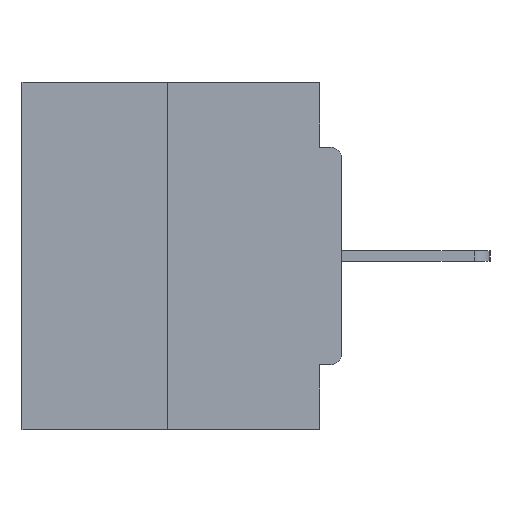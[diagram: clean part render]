
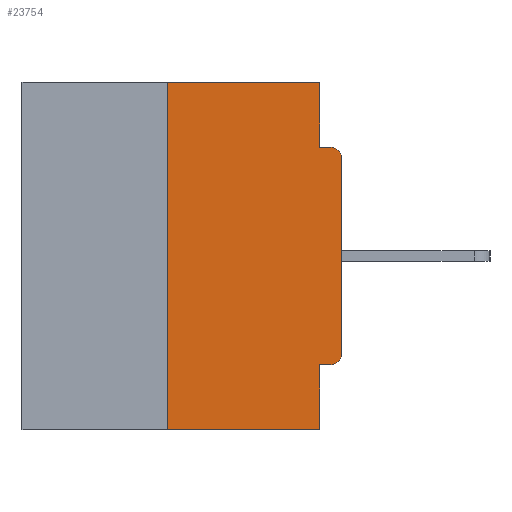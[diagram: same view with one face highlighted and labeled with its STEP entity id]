
A CAD part, left-side view. The second image highlights one B-rep face of the part: STEP entity #23754.
In plain terms, the highlighted planar face has unit normal (-1, 0, 0).
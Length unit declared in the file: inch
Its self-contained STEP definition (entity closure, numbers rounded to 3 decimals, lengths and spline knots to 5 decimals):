
#402 = VERTEX_POINT ( 'NONE', #31273 ) ;
#1106 = LINE ( 'NONE', #25379, #15881 ) ;
#1269 = VECTOR ( 'NONE', #26337, 39.37008 ) ;
#1753 = VERTEX_POINT ( 'NONE', #14833 ) ;
#2155 = VECTOR ( 'NONE', #20694, 39.37008 ) ;
#2261 = AXIS2_PLACEMENT_3D ( 'NONE', #11669, #24224, #5452 ) ;
#4445 = CARTESIAN_POINT ( 'NONE',  ( 0., 0., 0. ) ) ;
#5279 = CARTESIAN_POINT ( 'NONE',  ( 0., 0., -0.3915 ) ) ;
#5452 = DIRECTION ( 'NONE',  ( 0., 0., -1. ) ) ;
#5919 = EDGE_CURVE ( 'NONE', #8940, #1753, #33247, .T. ) ;
#6620 = DIRECTION ( 'NONE',  ( 0., 0., -1. ) ) ;
#6693 = CARTESIAN_POINT ( 'NONE',  ( 0., 0.015, -0.1085 ) ) ;
#6732 = ORIENTED_EDGE ( 'NONE', *, *, #8982, .T. ) ;
#8554 = VERTEX_POINT ( 'NONE', #39500 ) ;
#8940 = VERTEX_POINT ( 'NONE', #19826 ) ;
#8982 = EDGE_CURVE ( 'NONE', #19661, #14767, #25337, .T. ) ;
#9300 = VECTOR ( 'NONE', #33938, 39.37008 ) ;
#9754 = CARTESIAN_POINT ( 'NONE',  ( 0., 0., -0.1085 ) ) ;
#9851 = DIRECTION ( 'NONE',  ( 0., 0., -1. ) ) ;
#10511 = CARTESIAN_POINT ( 'NONE',  ( 0., 0.015, -0.0935 ) ) ;
#11559 = AXIS2_PLACEMENT_3D ( 'NONE', #17037, #38609, #20170 ) ;
#11669 = CARTESIAN_POINT ( 'NONE',  ( 0., 0.46, 0. ) ) ;
#12365 = CARTESIAN_POINT ( 'NONE',  ( 0., 0.46, -0.5 ) ) ;
#13371 = LINE ( 'NONE', #34215, #20705 ) ;
#14767 = VERTEX_POINT ( 'NONE', #9754 ) ;
#14833 = CARTESIAN_POINT ( 'NONE',  ( 0., 0.031, -0.5 ) ) ;
#15376 = DIRECTION ( 'NONE',  ( 0., -1., 0. ) ) ;
#15881 = VECTOR ( 'NONE', #6620, 39.37008 ) ;
#17037 = CARTESIAN_POINT ( 'NONE',  ( 0., 0.015, -0.3915 ) ) ;
#17578 = CARTESIAN_POINT ( 'NONE',  ( 0., 0., -0.4065 ) ) ;
#19661 = VERTEX_POINT ( 'NONE', #5279 ) ;
#19826 = CARTESIAN_POINT ( 'NONE',  ( 0., 0.031, -0.4065 ) ) ;
#20170 = DIRECTION ( 'NONE',  ( 0., 0., -1. ) ) ;
#20490 = VECTOR ( 'NONE', #21848, 39.37008 ) ;
#20694 = DIRECTION ( 'NONE',  ( 0., 1., 0. ) ) ;
#20705 = VECTOR ( 'NONE', #21890, 39.37008 ) ;
#21716 = ORIENTED_EDGE ( 'NONE', *, *, #23352, .F. ) ;
#21848 = DIRECTION ( 'NONE',  ( 0., 0., -1. ) ) ;
#21890 = DIRECTION ( 'NONE',  ( 0., -1., 0. ) ) ;
#22040 = ORIENTED_EDGE ( 'NONE', *, *, #30356, .F. ) ;
#22566 = ORIENTED_EDGE ( 'NONE', *, *, #37879, .T. ) ;
#22876 = LINE ( 'NONE', #34793, #38276 ) ;
#23080 = ORIENTED_EDGE ( 'NONE', *, *, #5919, .F. ) ;
#23352 = EDGE_CURVE ( 'NONE', #402, #8554, #22876, .T. ) ;
#23379 = ORIENTED_EDGE ( 'NONE', *, *, #26180, .T. ) ;
#23754 = ADVANCED_FACE ( 'NONE', ( #40130 ), #39527, .F. ) ;
#23858 = VECTOR ( 'NONE', #15376, 39.37008 ) ;
#24168 = VERTEX_POINT ( 'NONE', #38829 ) ;
#24224 = DIRECTION ( 'NONE',  ( 1., 0., 0. ) ) ;
#24860 = ORIENTED_EDGE ( 'NONE', *, *, #25760, .T. ) ;
#25337 = LINE ( 'NONE', #4445, #1269 ) ;
#25379 = CARTESIAN_POINT ( 'NONE',  ( 0., 0.031, 0. ) ) ;
#25760 = EDGE_CURVE ( 'NONE', #24168, #19661, #38092, .T. ) ;
#26069 = CIRCLE ( 'NONE', #33727, 0.015 ) ;
#26111 = EDGE_CURVE ( 'NONE', #35711, #40118, #13371, .T. ) ;
#26180 = EDGE_CURVE ( 'NONE', #14767, #40118, #26069, .T. ) ;
#26337 = DIRECTION ( 'NONE',  ( 0., 0., 1. ) ) ;
#26471 = CARTESIAN_POINT ( 'NONE',  ( 0., 0.25, -0.5 ) ) ;
#26864 = VERTEX_POINT ( 'NONE', #26471 ) ;
#27866 = LINE ( 'NONE', #30844, #9300 ) ;
#28027 = ORIENTED_EDGE ( 'NONE', *, *, #26111, .F. ) ;
#28565 = DIRECTION ( 'NONE',  ( -1., 0., 0. ) ) ;
#28619 = DIRECTION ( 'NONE',  ( 0., -1., 0. ) ) ;
#29087 = ORIENTED_EDGE ( 'NONE', *, *, #36549, .F. ) ;
#29676 = CARTESIAN_POINT ( 'NONE',  ( 0., 0.031, -0.0935 ) ) ;
#30356 = EDGE_CURVE ( 'NONE', #24168, #8940, #33422, .T. ) ;
#30844 = CARTESIAN_POINT ( 'NONE',  ( 0., 0.25, 0. ) ) ;
#31273 = CARTESIAN_POINT ( 'NONE',  ( 0., 0.25, 0. ) ) ;
#33247 = LINE ( 'NONE', #37211, #20490 ) ;
#33422 = LINE ( 'NONE', #17578, #2155 ) ;
#33727 = AXIS2_PLACEMENT_3D ( 'NONE', #6693, #28565, #9851 ) ;
#33938 = DIRECTION ( 'NONE',  ( 0., 0., 1. ) ) ;
#34215 = CARTESIAN_POINT ( 'NONE',  ( 0., 0., -0.0935 ) ) ;
#34494 = EDGE_CURVE ( 'NONE', #8554, #35711, #1106, .T. ) ;
#34793 = CARTESIAN_POINT ( 'NONE',  ( 0., 0.46, 0. ) ) ;
#35711 = VERTEX_POINT ( 'NONE', #29676 ) ;
#36549 = EDGE_CURVE ( 'NONE', #26864, #402, #27866, .T. ) ;
#37211 = CARTESIAN_POINT ( 'NONE',  ( 0., 0.031, -0.5 ) ) ;
#37624 = ORIENTED_EDGE ( 'NONE', *, *, #34494, .F. ) ;
#37879 = EDGE_CURVE ( 'NONE', #26864, #1753, #40179, .T. ) ;
#38092 = CIRCLE ( 'NONE', #11559, 0.015 ) ;
#38276 = VECTOR ( 'NONE', #28619, 39.37008 ) ;
#38609 = DIRECTION ( 'NONE',  ( -1., 0., 0. ) ) ;
#38829 = CARTESIAN_POINT ( 'NONE',  ( 0., 0.015, -0.4065 ) ) ;
#39500 = CARTESIAN_POINT ( 'NONE',  ( 0., 0.031, 0. ) ) ;
#39527 = PLANE ( 'NONE',  #2261 ) ;
#39721 = EDGE_LOOP ( 'NONE', ( #21716, #29087, #22566, #23080, #22040, #24860, #6732, #23379, #28027, #37624 ) ) ;
#40118 = VERTEX_POINT ( 'NONE', #10511 ) ;
#40130 = FACE_OUTER_BOUND ( 'NONE', #39721, .T. ) ;
#40179 = LINE ( 'NONE', #12365, #23858 ) ;
